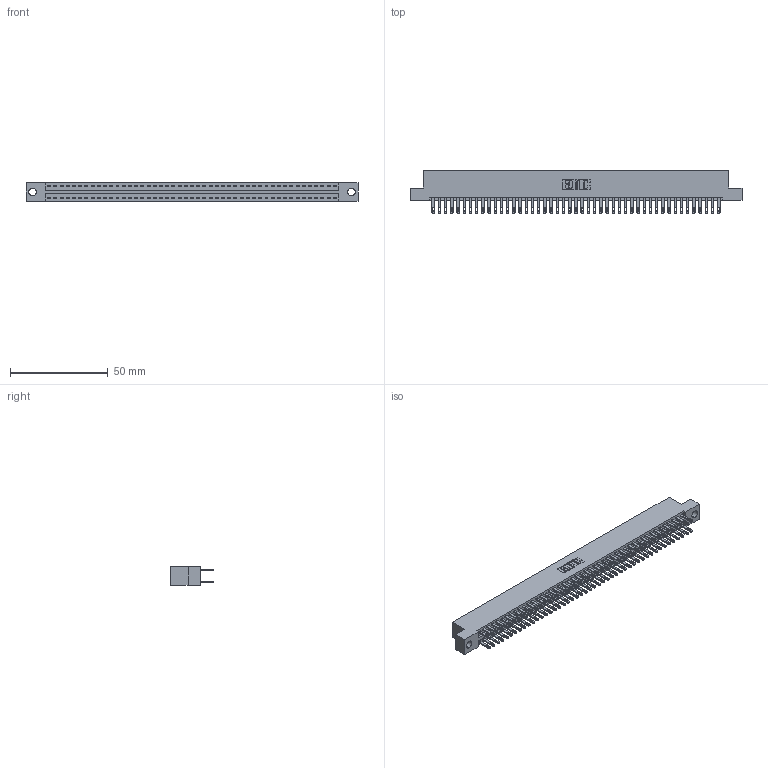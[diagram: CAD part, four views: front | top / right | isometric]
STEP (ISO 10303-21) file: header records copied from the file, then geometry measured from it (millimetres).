
FILE_DESCRIPTION (( 'STEP AP203' ), '1' );
FILE_NAME ('346-094-500-204.STEP', '2022-05-26T09:03:15', ( '' ), ( '' ), 'SwSTEP 2.0', 'SolidWorks 2020', '' );
FILE_SCHEMA (( 'CONFIG_CONTROL_DESIGN' ));
Length unit declared in the file: inch
Products named in the file (3): 345-292-001_345-293-100; 346 Part_Flush Mounting Lugs - 0.156 Dia-TH; 346-094-500-204
Assembly tree (95 placements, depth 2):
  346-094-500-204
    346 Part_Flush Mounting Lugs - 0.156 Dia-TH
    345-292-001_345-293-100  x94
Bounding box: 169.8 x 21.84 x 9.4 mm (x, y, z)
Volume: 16777.6 mm3; surface area: 23972.3 mm2
Topology: 95 solids, 95 shells, 4648 faces, 14183 edges, 9454 vertices
Faces by surface type: plane 2816, cylinder 1832
Entity records: 30349 total; most frequent: CARTESIAN_POINT 4998, ORIENTED_EDGE 4930, DIRECTION 4457, EDGE_CURVE 2465, VECTOR 2141, LINE 2141, VERTEX_POINT 1642, AXIS2_PLACEMENT_3D 1158
